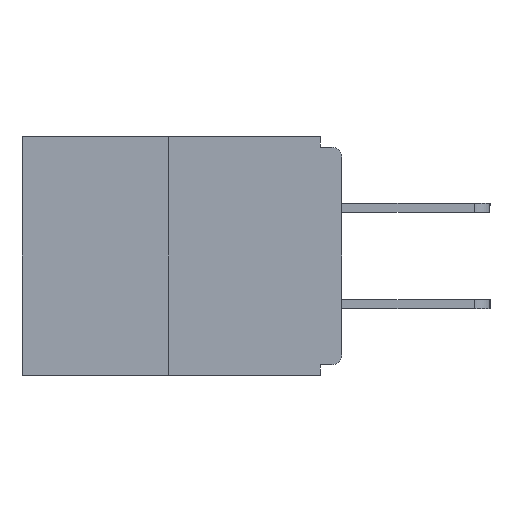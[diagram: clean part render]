
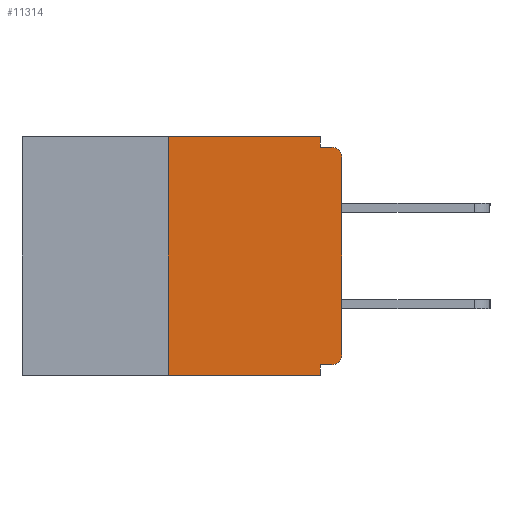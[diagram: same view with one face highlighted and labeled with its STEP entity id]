
A CAD part, left-side view. The second image highlights one B-rep face of the part: STEP entity #11314.
In plain terms, the highlighted planar face has unit normal (-1, 0, 0).
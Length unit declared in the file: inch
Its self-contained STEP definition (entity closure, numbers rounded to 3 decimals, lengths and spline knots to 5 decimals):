
#409 = CARTESIAN_POINT ( 'NONE',  ( 0., 0., -0.313 ) ) ;
#538 = DIRECTION ( 'NONE',  ( 0., 0., 1. ) ) ;
#773 = DIRECTION ( 'NONE',  ( 0., 0., -1. ) ) ;
#1009 = CARTESIAN_POINT ( 'NONE',  ( 0., 0.031, -0.343 ) ) ;
#1437 = EDGE_CURVE ( 'NONE', #16000, #13837, #15225, .T. ) ;
#1616 = ORIENTED_EDGE ( 'NONE', *, *, #4415, .F. ) ;
#1764 = EDGE_CURVE ( 'NONE', #16985, #9844, #5457, .T. ) ;
#1874 = ORIENTED_EDGE ( 'NONE', *, *, #15272, .T. ) ;
#1960 = ORIENTED_EDGE ( 'NONE', *, *, #1437, .F. ) ;
#1986 = CARTESIAN_POINT ( 'NONE',  ( 0., 0.031, -0.343 ) ) ;
#1999 = LINE ( 'NONE', #6695, #11998 ) ;
#2118 = CARTESIAN_POINT ( 'NONE',  ( 0., 0.25, 0. ) ) ;
#2170 = CARTESIAN_POINT ( 'NONE',  ( 0., 0.46, 0. ) ) ;
#2804 = DIRECTION ( 'NONE',  ( 0., -1., 0. ) ) ;
#3170 = AXIS2_PLACEMENT_3D ( 'NONE', #12896, #22696, #6937 ) ;
#3287 = VECTOR ( 'NONE', #9390, 39.37008 ) ;
#3454 = LINE ( 'NONE', #2170, #17128 ) ;
#3543 = LINE ( 'NONE', #2118, #17845 ) ;
#4415 = EDGE_CURVE ( 'NONE', #15086, #12895, #3543, .T. ) ;
#4611 = CARTESIAN_POINT ( 'NONE',  ( 0., 0.015, -0.015 ) ) ;
#4798 = DIRECTION ( 'NONE',  ( -1., 0., 0. ) ) ;
#5030 = CARTESIAN_POINT ( 'NONE',  ( 0., 0.031, 0. ) ) ;
#5066 = VERTEX_POINT ( 'NONE', #12105 ) ;
#5266 = CARTESIAN_POINT ( 'NONE',  ( 0., 0., -0.328 ) ) ;
#5389 = LINE ( 'NONE', #1009, #3287 ) ;
#5457 = LINE ( 'NONE', #11495, #22814 ) ;
#5864 = CARTESIAN_POINT ( 'NONE',  ( 0., 0., 0. ) ) ;
#6183 = ORIENTED_EDGE ( 'NONE', *, *, #1764, .F. ) ;
#6408 = EDGE_CURVE ( 'NONE', #13837, #20521, #5389, .T. ) ;
#6666 = ORIENTED_EDGE ( 'NONE', *, *, #17943, .T. ) ;
#6683 = ORIENTED_EDGE ( 'NONE', *, *, #21437, .T. ) ;
#6695 = CARTESIAN_POINT ( 'NONE',  ( 0., 0.031, 0. ) ) ;
#6937 = DIRECTION ( 'NONE',  ( 0., 0., -1. ) ) ;
#7237 = CARTESIAN_POINT ( 'NONE',  ( 0., 0.031, -0.328 ) ) ;
#7585 = FACE_OUTER_BOUND ( 'NONE', #10868, .T. ) ;
#8080 = CARTESIAN_POINT ( 'NONE',  ( 0., 0.031, -0.015 ) ) ;
#8096 = DIRECTION ( 'NONE',  ( 0., -1., 0. ) ) ;
#8141 = CARTESIAN_POINT ( 'NONE',  ( 0., 0.015, -0.03 ) ) ;
#8279 = VECTOR ( 'NONE', #538, 39.37008 ) ;
#8417 = EDGE_CURVE ( 'NONE', #18972, #16985, #1999, .T. ) ;
#9181 = CARTESIAN_POINT ( 'NONE',  ( 0., 0.25, -0.343 ) ) ;
#9390 = DIRECTION ( 'NONE',  ( 0., 0., -1. ) ) ;
#9501 = CIRCLE ( 'NONE', #22576, 0.015 ) ;
#9610 = EDGE_CURVE ( 'NONE', #12895, #18972, #3454, .T. ) ;
#9844 = VERTEX_POINT ( 'NONE', #4611 ) ;
#9989 = CIRCLE ( 'NONE', #17581, 0.015 ) ;
#10868 = EDGE_LOOP ( 'NONE', ( #19007, #1616, #6666, #25020, #1960, #6683, #13866, #1874, #6183, #22550 ) ) ;
#11152 = CARTESIAN_POINT ( 'NONE',  ( 0., 0.25, 0. ) ) ;
#11314 = ADVANCED_FACE ( 'NONE', ( #7585 ), #20481, .F. ) ;
#11495 = CARTESIAN_POINT ( 'NONE',  ( 0., 0., -0.015 ) ) ;
#11998 = VECTOR ( 'NONE', #773, 39.37008 ) ;
#12105 = CARTESIAN_POINT ( 'NONE',  ( 0., 0., -0.03 ) ) ;
#12201 = EDGE_CURVE ( 'NONE', #19661, #5066, #19568, .T. ) ;
#12309 = DIRECTION ( 'NONE',  ( 0., 0., -1. ) ) ;
#12895 = VERTEX_POINT ( 'NONE', #11152 ) ;
#12896 = CARTESIAN_POINT ( 'NONE',  ( 0., 0.46, 0. ) ) ;
#13837 = VERTEX_POINT ( 'NONE', #7237 ) ;
#13843 = DIRECTION ( 'NONE',  ( 0., 0., 1. ) ) ;
#13866 = ORIENTED_EDGE ( 'NONE', *, *, #12201, .T. ) ;
#14006 = DIRECTION ( 'NONE',  ( -1., 0., 0. ) ) ;
#15086 = VERTEX_POINT ( 'NONE', #9181 ) ;
#15225 = LINE ( 'NONE', #5266, #17680 ) ;
#15258 = DIRECTION ( 'NONE',  ( 0., -1., 0. ) ) ;
#15272 = EDGE_CURVE ( 'NONE', #5066, #9844, #9989, .T. ) ;
#16000 = VERTEX_POINT ( 'NONE', #16976 ) ;
#16796 = CARTESIAN_POINT ( 'NONE',  ( 0., 0.015, -0.313 ) ) ;
#16976 = CARTESIAN_POINT ( 'NONE',  ( 0., 0.015, -0.328 ) ) ;
#16985 = VERTEX_POINT ( 'NONE', #8080 ) ;
#17128 = VECTOR ( 'NONE', #8096, 39.37008 ) ;
#17581 = AXIS2_PLACEMENT_3D ( 'NONE', #8141, #14006, #12309 ) ;
#17680 = VECTOR ( 'NONE', #18872, 39.37008 ) ;
#17845 = VECTOR ( 'NONE', #13843, 39.37008 ) ;
#17943 = EDGE_CURVE ( 'NONE', #15086, #20521, #23587, .T. ) ;
#18422 = DIRECTION ( 'NONE',  ( 0., 0., -1. ) ) ;
#18872 = DIRECTION ( 'NONE',  ( 0., 1., 0. ) ) ;
#18972 = VERTEX_POINT ( 'NONE', #5030 ) ;
#19007 = ORIENTED_EDGE ( 'NONE', *, *, #9610, .F. ) ;
#19568 = LINE ( 'NONE', #5864, #8279 ) ;
#19661 = VERTEX_POINT ( 'NONE', #409 ) ;
#20481 = PLANE ( 'NONE',  #3170 ) ;
#20521 = VERTEX_POINT ( 'NONE', #1986 ) ;
#21437 = EDGE_CURVE ( 'NONE', #16000, #19661, #9501, .T. ) ;
#22550 = ORIENTED_EDGE ( 'NONE', *, *, #8417, .F. ) ;
#22576 = AXIS2_PLACEMENT_3D ( 'NONE', #16796, #4798, #18422 ) ;
#22696 = DIRECTION ( 'NONE',  ( 1., 0., 0. ) ) ;
#22814 = VECTOR ( 'NONE', #15258, 39.37008 ) ;
#23273 = VECTOR ( 'NONE', #2804, 39.37008 ) ;
#23587 = LINE ( 'NONE', #23793, #23273 ) ;
#23793 = CARTESIAN_POINT ( 'NONE',  ( 0., 0.46, -0.343 ) ) ;
#25020 = ORIENTED_EDGE ( 'NONE', *, *, #6408, .F. ) ;
